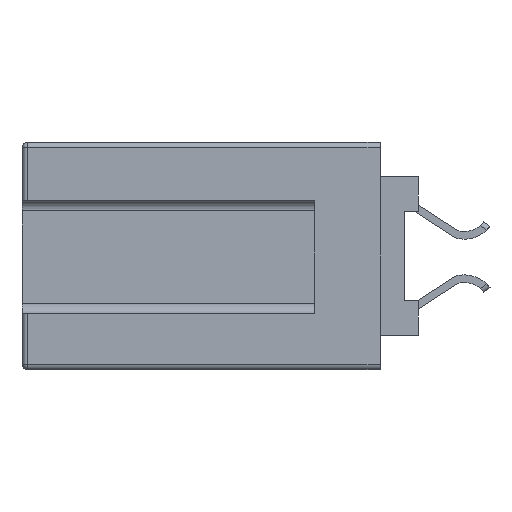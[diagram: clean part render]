
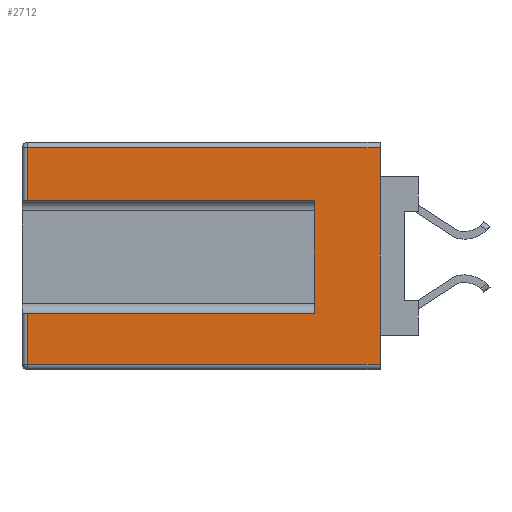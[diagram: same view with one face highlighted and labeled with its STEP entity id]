
A CAD part, left-side view. The second image highlights one B-rep face of the part: STEP entity #2712.
In plain terms, the highlighted planar face has unit normal (-1, 0, 0).
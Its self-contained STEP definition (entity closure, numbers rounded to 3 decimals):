
#2184 = VECTOR ( 'NONE', #29652, 1000. ) ;
#2712 = ADVANCED_FACE ( 'NONE', ( #10664 ), #20692, .F. ) ;
#2927 = DIRECTION ( 'NONE',  ( 1., 0., 0. ) ) ;
#3777 = DIRECTION ( 'NONE',  ( 0., 0., -1. ) ) ;
#6151 = VECTOR ( 'NONE', #34617, 1000. ) ;
#8328 = DIRECTION ( 'NONE',  ( 0., 0., -1. ) ) ;
#8537 = CARTESIAN_POINT ( 'NONE',  ( 0., 4.07, -2.28 ) ) ;
#9099 = CARTESIAN_POINT ( 'NONE',  ( 0., 15.5, -8.68 ) ) ;
#9336 = ORIENTED_EDGE ( 'NONE', *, *, #11356, .T. ) ;
#9345 = LINE ( 'NONE', #23207, #37190 ) ;
#10664 = FACE_OUTER_BOUND ( 'NONE', #42480, .T. ) ;
#11356 = EDGE_CURVE ( 'NONE', #32934, #19937, #29477, .T. ) ;
#11481 = EDGE_CURVE ( 'NONE', #26396, #26741, #17097, .T. ) ;
#12931 = LINE ( 'NONE', #9099, #40093 ) ;
#13707 = VECTOR ( 'NONE', #14841, 1000. ) ;
#14500 = ORIENTED_EDGE ( 'NONE', *, *, #40677, .T. ) ;
#14670 = EDGE_CURVE ( 'NONE', #19937, #31615, #19371, .T. ) ;
#14841 = DIRECTION ( 'NONE',  ( 0., 1., 0. ) ) ;
#16133 = VERTEX_POINT ( 'NONE', #16645 ) ;
#16148 = EDGE_CURVE ( 'NONE', #40663, #32934, #20087, .T. ) ;
#16606 = ORIENTED_EDGE ( 'NONE', *, *, #11481, .F. ) ;
#16645 = CARTESIAN_POINT ( 'NONE',  ( 0., 15.3, -0.2 ) ) ;
#16974 = CARTESIAN_POINT ( 'NONE',  ( 0., 15.3, -2.28 ) ) ;
#17097 = LINE ( 'NONE', #34391, #6151 ) ;
#17847 = EDGE_CURVE ( 'NONE', #16133, #40663, #9345, .T. ) ;
#19371 = LINE ( 'NONE', #36430, #13707 ) ;
#19937 = VERTEX_POINT ( 'NONE', #26694 ) ;
#19984 = EDGE_CURVE ( 'NONE', #26396, #16133, #44415, .T. ) ;
#20087 = LINE ( 'NONE', #27345, #27608 ) ;
#20692 = PLANE ( 'NONE',  #24829 ) ;
#20861 = CARTESIAN_POINT ( 'NONE',  ( 0., 4.07, -2.28 ) ) ;
#22280 = EDGE_CURVE ( 'NONE', #32927, #26741, #12931, .T. ) ;
#23097 = ORIENTED_EDGE ( 'NONE', *, *, #22280, .T. ) ;
#23207 = CARTESIAN_POINT ( 'NONE',  ( 0., 15.3, 0. ) ) ;
#24469 = LINE ( 'NONE', #38132, #28660 ) ;
#24829 = AXIS2_PLACEMENT_3D ( 'NONE', #27051, #2927, #40939 ) ;
#26396 = VERTEX_POINT ( 'NONE', #33363 ) ;
#26694 = CARTESIAN_POINT ( 'NONE',  ( 0., 4.07, -6.68 ) ) ;
#26741 = VERTEX_POINT ( 'NONE', #31740 ) ;
#27051 = CARTESIAN_POINT ( 'NONE',  ( 0., 15.5, 0. ) ) ;
#27345 = CARTESIAN_POINT ( 'NONE',  ( 0., 4.07, -2.28 ) ) ;
#27608 = VECTOR ( 'NONE', #41217, 1000. ) ;
#28234 = CARTESIAN_POINT ( 'NONE',  ( 0., 15.3, -6.68 ) ) ;
#28660 = VECTOR ( 'NONE', #3777, 1000. ) ;
#29477 = LINE ( 'NONE', #8537, #33754 ) ;
#29556 = DIRECTION ( 'NONE',  ( 0., -1., 0. ) ) ;
#29652 = DIRECTION ( 'NONE',  ( 0., 1., 0. ) ) ;
#30860 = ORIENTED_EDGE ( 'NONE', *, *, #14670, .T. ) ;
#31615 = VERTEX_POINT ( 'NONE', #28234 ) ;
#31740 = CARTESIAN_POINT ( 'NONE',  ( 0., 1.5, -8.68 ) ) ;
#32927 = VERTEX_POINT ( 'NONE', #41555 ) ;
#32934 = VERTEX_POINT ( 'NONE', #20861 ) ;
#33363 = CARTESIAN_POINT ( 'NONE',  ( 0., 1.5, -0.2 ) ) ;
#33754 = VECTOR ( 'NONE', #8328, 1000. ) ;
#34317 = ORIENTED_EDGE ( 'NONE', *, *, #16148, .T. ) ;
#34391 = CARTESIAN_POINT ( 'NONE',  ( 0., 1.5, 0. ) ) ;
#34529 = ORIENTED_EDGE ( 'NONE', *, *, #17847, .T. ) ;
#34617 = DIRECTION ( 'NONE',  ( 0., 0., -1. ) ) ;
#36430 = CARTESIAN_POINT ( 'NONE',  ( 0., 4.07, -6.68 ) ) ;
#36493 = CARTESIAN_POINT ( 'NONE',  ( 0., 15.5, -0.2 ) ) ;
#37096 = DIRECTION ( 'NONE',  ( 0., 0., -1. ) ) ;
#37190 = VECTOR ( 'NONE', #37096, 1000. ) ;
#38132 = CARTESIAN_POINT ( 'NONE',  ( 0., 15.3, 0. ) ) ;
#39906 = ORIENTED_EDGE ( 'NONE', *, *, #19984, .T. ) ;
#40093 = VECTOR ( 'NONE', #29556, 1000. ) ;
#40663 = VERTEX_POINT ( 'NONE', #16974 ) ;
#40677 = EDGE_CURVE ( 'NONE', #31615, #32927, #24469, .T. ) ;
#40939 = DIRECTION ( 'NONE',  ( 0., 0., -1. ) ) ;
#41217 = DIRECTION ( 'NONE',  ( 0., -1., 0. ) ) ;
#41555 = CARTESIAN_POINT ( 'NONE',  ( 0., 15.3, -8.68 ) ) ;
#42480 = EDGE_LOOP ( 'NONE', ( #14500, #23097, #16606, #39906, #34529, #34317, #9336, #30860 ) ) ;
#44415 = LINE ( 'NONE', #36493, #2184 ) ;
